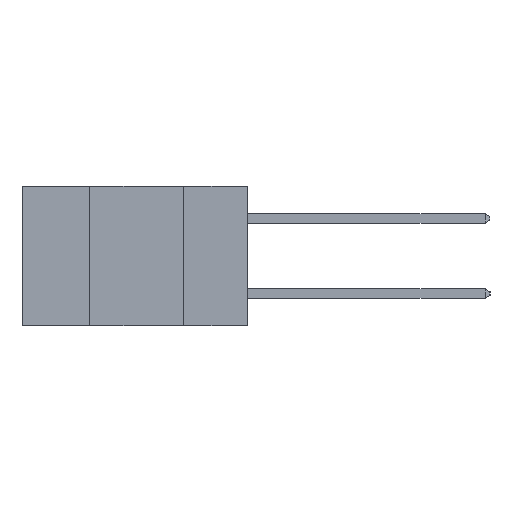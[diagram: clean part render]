
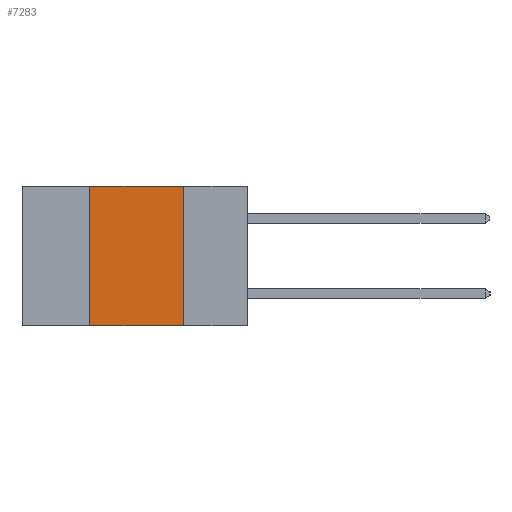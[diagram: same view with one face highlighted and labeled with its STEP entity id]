
A CAD part, left-side view. The second image highlights one B-rep face of the part: STEP entity #7283.
In plain terms, the highlighted planar face has unit normal (-1, 0, 0).
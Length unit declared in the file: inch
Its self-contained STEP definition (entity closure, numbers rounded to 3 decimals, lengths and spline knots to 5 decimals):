
#932 = VECTOR ( 'NONE', #19024, 39.37008 ) ;
#1235 = DIRECTION ( 'NONE',  ( 0., 0., -1. ) ) ;
#1387 = CARTESIAN_POINT ( 'NONE',  ( 0., 0.6, -0.37 ) ) ;
#1668 = VERTEX_POINT ( 'NONE', #2101 ) ;
#2101 = CARTESIAN_POINT ( 'NONE',  ( 0., 0.42, 0. ) ) ;
#2837 = LINE ( 'NONE', #19634, #18768 ) ;
#3056 = ORIENTED_EDGE ( 'NONE', *, *, #6943, .F. ) ;
#3079 = ORIENTED_EDGE ( 'NONE', *, *, #10875, .F. ) ;
#4640 = AXIS2_PLACEMENT_3D ( 'NONE', #9082, #10655, #1235 ) ;
#5070 = VERTEX_POINT ( 'NONE', #7046 ) ;
#5584 = VERTEX_POINT ( 'NONE', #17350 ) ;
#6534 = VECTOR ( 'NONE', #13857, 39.37008 ) ;
#6943 = EDGE_CURVE ( 'NONE', #10085, #5070, #13373, .T. ) ;
#7046 = CARTESIAN_POINT ( 'NONE',  ( 0., 0.17, -0.37 ) ) ;
#7283 = ADVANCED_FACE ( 'NONE', ( #16421 ), #7503, .F. ) ;
#7503 = PLANE ( 'NONE',  #4640 ) ;
#8134 = CARTESIAN_POINT ( 'NONE',  ( 0., 0.42, -0.37 ) ) ;
#8335 = CARTESIAN_POINT ( 'NONE',  ( 0., 0.17, -0.37 ) ) ;
#8798 = EDGE_CURVE ( 'NONE', #5584, #5070, #10715, .T. ) ;
#9082 = CARTESIAN_POINT ( 'NONE',  ( 0., 0.6, 0. ) ) ;
#10085 = VERTEX_POINT ( 'NONE', #17136 ) ;
#10383 = LINE ( 'NONE', #8134, #18937 ) ;
#10655 = DIRECTION ( 'NONE',  ( 1., 0., 0. ) ) ;
#10715 = LINE ( 'NONE', #1387, #6534 ) ;
#10875 = EDGE_CURVE ( 'NONE', #5584, #1668, #10383, .T. ) ;
#10912 = ORIENTED_EDGE ( 'NONE', *, *, #18096, .F. ) ;
#13373 = LINE ( 'NONE', #8335, #932 ) ;
#13614 = DIRECTION ( 'NONE',  ( 0., -1., 0. ) ) ;
#13857 = DIRECTION ( 'NONE',  ( 0., -1., 0. ) ) ;
#14508 = ORIENTED_EDGE ( 'NONE', *, *, #8798, .T. ) ;
#16421 = FACE_OUTER_BOUND ( 'NONE', #18615, .T. ) ;
#17136 = CARTESIAN_POINT ( 'NONE',  ( 0., 0.17, 0. ) ) ;
#17350 = CARTESIAN_POINT ( 'NONE',  ( 0., 0.42, -0.37 ) ) ;
#18096 = EDGE_CURVE ( 'NONE', #1668, #10085, #2837, .T. ) ;
#18615 = EDGE_LOOP ( 'NONE', ( #3056, #10912, #3079, #14508 ) ) ;
#18768 = VECTOR ( 'NONE', #13614, 39.37008 ) ;
#18819 = DIRECTION ( 'NONE',  ( 0., 0., 1. ) ) ;
#18937 = VECTOR ( 'NONE', #18819, 39.37008 ) ;
#19024 = DIRECTION ( 'NONE',  ( 0., 0., -1. ) ) ;
#19634 = CARTESIAN_POINT ( 'NONE',  ( 0., 0.6, 0. ) ) ;
